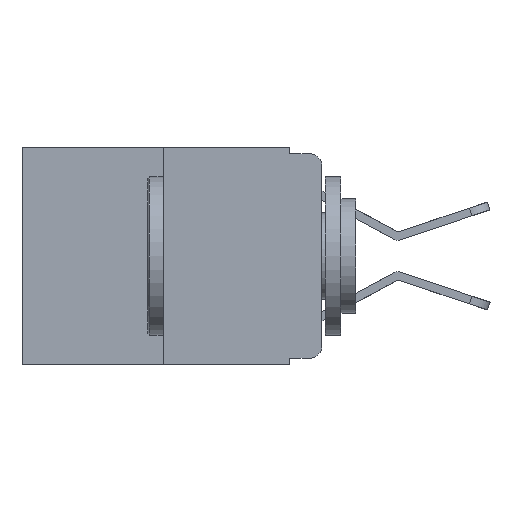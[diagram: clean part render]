
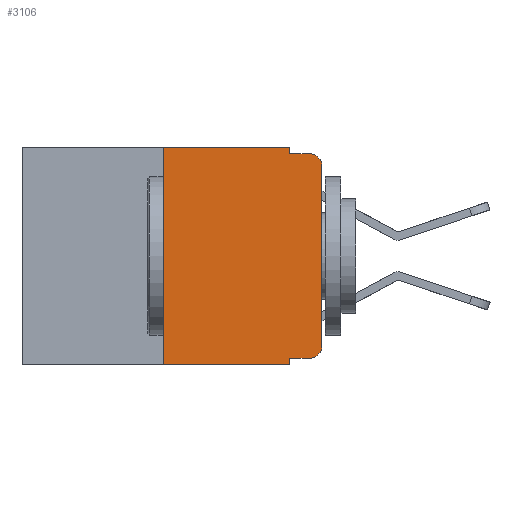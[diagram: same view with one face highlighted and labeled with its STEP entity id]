
A CAD part, left-side view. The second image highlights one B-rep face of the part: STEP entity #3106.
In plain terms, the highlighted planar face has unit normal (-1, 0, 0).
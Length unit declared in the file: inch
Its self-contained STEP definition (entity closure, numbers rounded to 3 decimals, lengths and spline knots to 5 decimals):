
#162 = VERTEX_POINT ( 'NONE', #10707 ) ;
#406 = CARTESIAN_POINT ( 'NONE',  ( 0., 0.02, -0.333 ) ) ;
#745 = EDGE_LOOP ( 'NONE', ( #7767, #2224, #12569, #16977, #9466, #2579, #8046, #13625, #952, #15707 ) ) ;
#912 = CARTESIAN_POINT ( 'NONE',  ( 0., 0.473, -0.343 ) ) ;
#952 = ORIENTED_EDGE ( 'NONE', *, *, #8408, .T. ) ;
#1035 = LINE ( 'NONE', #912, #11297 ) ;
#2224 = ORIENTED_EDGE ( 'NONE', *, *, #18026, .T. ) ;
#2465 = VERTEX_POINT ( 'NONE', #9678 ) ;
#2531 = CARTESIAN_POINT ( 'NONE',  ( 0., 0.051, 0. ) ) ;
#2579 = ORIENTED_EDGE ( 'NONE', *, *, #21038, .F. ) ;
#3043 = VERTEX_POINT ( 'NONE', #8932 ) ;
#3105 = LINE ( 'NONE', #3225, #5958 ) ;
#3106 = ADVANCED_FACE ( 'NONE', ( #16441 ), #7972, .F. ) ;
#3225 = CARTESIAN_POINT ( 'NONE',  ( 0., 0.473, 0. ) ) ;
#4163 = LINE ( 'NONE', #2531, #11489 ) ;
#4230 = VERTEX_POINT ( 'NONE', #7482 ) ;
#4248 = EDGE_CURVE ( 'NONE', #9153, #17063, #16635, .T. ) ;
#4392 = VECTOR ( 'NONE', #12997, 39.37008 ) ;
#4443 = VECTOR ( 'NONE', #8930, 39.37008 ) ;
#4626 = DIRECTION ( 'NONE',  ( 0., 0., -1. ) ) ;
#4887 = DIRECTION ( 'NONE',  ( 0., 0., 1. ) ) ;
#4944 = CARTESIAN_POINT ( 'NONE',  ( 0., 0.02, -0.03 ) ) ;
#5473 = CARTESIAN_POINT ( 'NONE',  ( 0., 0.051, -0.333 ) ) ;
#5845 = VERTEX_POINT ( 'NONE', #20632 ) ;
#5902 = LINE ( 'NONE', #11237, #4392 ) ;
#5958 = VECTOR ( 'NONE', #22363, 39.37008 ) ;
#5961 = AXIS2_PLACEMENT_3D ( 'NONE', #9738, #18211, #16792 ) ;
#6106 = CARTESIAN_POINT ( 'NONE',  ( 0., 0.051, 0. ) ) ;
#6138 = LINE ( 'NONE', #17242, #13839 ) ;
#6774 = DIRECTION ( 'NONE',  ( 0., 0., -1. ) ) ;
#7276 = EDGE_CURVE ( 'NONE', #4230, #2465, #5902, .T. ) ;
#7407 = LINE ( 'NONE', #15896, #4443 ) ;
#7482 = CARTESIAN_POINT ( 'NONE',  ( 0., 0.051, -0.01 ) ) ;
#7767 = ORIENTED_EDGE ( 'NONE', *, *, #13783, .T. ) ;
#7972 = PLANE ( 'NONE',  #5961 ) ;
#8046 = ORIENTED_EDGE ( 'NONE', *, *, #17273, .T. ) ;
#8408 = EDGE_CURVE ( 'NONE', #9153, #21763, #7407, .T. ) ;
#8732 = AXIS2_PLACEMENT_3D ( 'NONE', #4944, #15263, #6774 ) ;
#8752 = VECTOR ( 'NONE', #4626, 39.37008 ) ;
#8930 = DIRECTION ( 'NONE',  ( 0., -1., 0. ) ) ;
#8932 = CARTESIAN_POINT ( 'NONE',  ( 0., 0., -0.313 ) ) ;
#8950 = EDGE_CURVE ( 'NONE', #162, #4230, #4163, .T. ) ;
#9153 = VERTEX_POINT ( 'NONE', #5473 ) ;
#9466 = ORIENTED_EDGE ( 'NONE', *, *, #10317, .F. ) ;
#9678 = CARTESIAN_POINT ( 'NONE',  ( 0., 0.02, -0.01 ) ) ;
#9738 = CARTESIAN_POINT ( 'NONE',  ( 0., 0.473, 0. ) ) ;
#10317 = EDGE_CURVE ( 'NONE', #13275, #162, #3105, .T. ) ;
#10707 = CARTESIAN_POINT ( 'NONE',  ( 0., 0.051, 0. ) ) ;
#11237 = CARTESIAN_POINT ( 'NONE',  ( 0., 0.051, -0.01 ) ) ;
#11297 = VECTOR ( 'NONE', #13422, 39.37008 ) ;
#11489 = VECTOR ( 'NONE', #18540, 39.37008 ) ;
#12242 = EDGE_CURVE ( 'NONE', #21763, #3043, #21618, .T. ) ;
#12569 = ORIENTED_EDGE ( 'NONE', *, *, #7276, .F. ) ;
#12828 = CARTESIAN_POINT ( 'NONE',  ( 0., 0.25, -0.343 ) ) ;
#12997 = DIRECTION ( 'NONE',  ( 0., -1., 0. ) ) ;
#13137 = VERTEX_POINT ( 'NONE', #12828 ) ;
#13275 = VERTEX_POINT ( 'NONE', #20241 ) ;
#13422 = DIRECTION ( 'NONE',  ( 0., -1., 0. ) ) ;
#13625 = ORIENTED_EDGE ( 'NONE', *, *, #4248, .F. ) ;
#13783 = EDGE_CURVE ( 'NONE', #3043, #5845, #6138, .T. ) ;
#13839 = VECTOR ( 'NONE', #4887, 39.37008 ) ;
#14071 = CARTESIAN_POINT ( 'NONE',  ( 0., 0.02, -0.313 ) ) ;
#14565 = AXIS2_PLACEMENT_3D ( 'NONE', #14071, #19533, #16131 ) ;
#15263 = DIRECTION ( 'NONE',  ( -1., 0., 0. ) ) ;
#15707 = ORIENTED_EDGE ( 'NONE', *, *, #12242, .T. ) ;
#15850 = CARTESIAN_POINT ( 'NONE',  ( 0., 0.051, -0.343 ) ) ;
#15896 = CARTESIAN_POINT ( 'NONE',  ( 0., 0.051, -0.333 ) ) ;
#16131 = DIRECTION ( 'NONE',  ( 0., 0., -1. ) ) ;
#16441 = FACE_OUTER_BOUND ( 'NONE', #745, .T. ) ;
#16479 = CIRCLE ( 'NONE', #8732, 0.02 ) ;
#16635 = LINE ( 'NONE', #6106, #8752 ) ;
#16792 = DIRECTION ( 'NONE',  ( 0., 0., -1. ) ) ;
#16922 = VECTOR ( 'NONE', #18949, 39.37008 ) ;
#16977 = ORIENTED_EDGE ( 'NONE', *, *, #8950, .F. ) ;
#17063 = VERTEX_POINT ( 'NONE', #15850 ) ;
#17242 = CARTESIAN_POINT ( 'NONE',  ( 0., 0., 0. ) ) ;
#17273 = EDGE_CURVE ( 'NONE', #13137, #17063, #1035, .T. ) ;
#18026 = EDGE_CURVE ( 'NONE', #5845, #2465, #16479, .T. ) ;
#18211 = DIRECTION ( 'NONE',  ( 1., 0., 0. ) ) ;
#18540 = DIRECTION ( 'NONE',  ( 0., 0., -1. ) ) ;
#18949 = DIRECTION ( 'NONE',  ( 0., 0., 1. ) ) ;
#19297 = LINE ( 'NONE', #22668, #16922 ) ;
#19533 = DIRECTION ( 'NONE',  ( -1., 0., 0. ) ) ;
#20241 = CARTESIAN_POINT ( 'NONE',  ( 0., 0.25, 0. ) ) ;
#20632 = CARTESIAN_POINT ( 'NONE',  ( 0., 0., -0.03 ) ) ;
#21038 = EDGE_CURVE ( 'NONE', #13137, #13275, #19297, .T. ) ;
#21618 = CIRCLE ( 'NONE', #14565, 0.02 ) ;
#21763 = VERTEX_POINT ( 'NONE', #406 ) ;
#22363 = DIRECTION ( 'NONE',  ( 0., -1., 0. ) ) ;
#22668 = CARTESIAN_POINT ( 'NONE',  ( 0., 0.25, 0. ) ) ;
